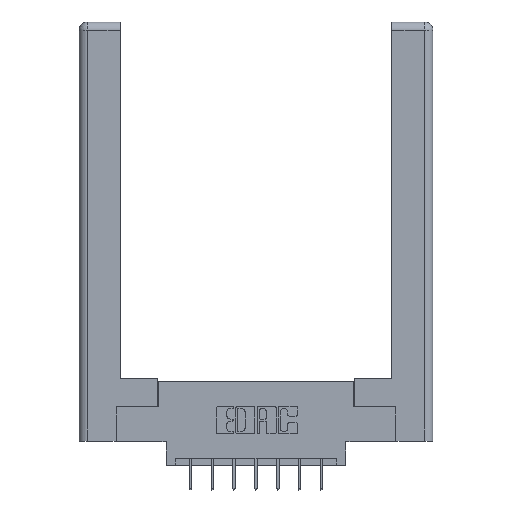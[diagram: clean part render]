
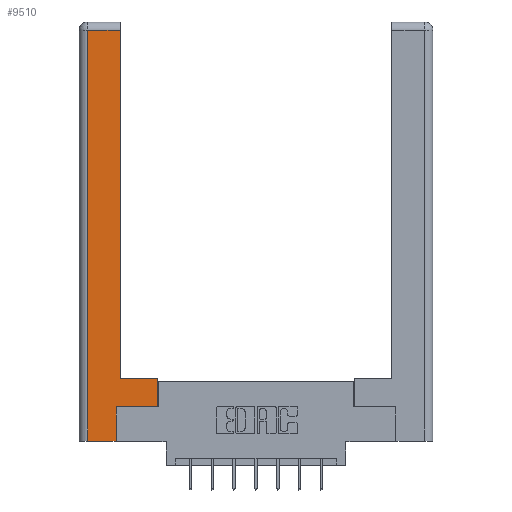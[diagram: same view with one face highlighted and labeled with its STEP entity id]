
A CAD part, top view. The second image highlights one B-rep face of the part: STEP entity #9510.
In plain terms, the highlighted planar face has unit normal (0, 0, 1).
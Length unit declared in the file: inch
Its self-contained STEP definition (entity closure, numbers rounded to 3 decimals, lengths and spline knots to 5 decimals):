
#22 = VECTOR ( 'NONE', #7003, 39.37008 ) ;
#182 = EDGE_CURVE ( 'NONE', #4637, #9045, #12069, .T. ) ;
#260 = EDGE_CURVE ( 'NONE', #9697, #6665, #2271, .T. ) ;
#274 = DIRECTION ( 'NONE',  ( 1., 0., 0. ) ) ;
#299 = DIRECTION ( 'NONE',  ( -1., 0., 0. ) ) ;
#448 = CARTESIAN_POINT ( 'NONE',  ( 0.265, 0., 0. ) ) ;
#798 = LINE ( 'NONE', #4582, #10724 ) ;
#1360 = EDGE_CURVE ( 'NONE', #6665, #6210, #3975, .T. ) ;
#1703 = CARTESIAN_POINT ( 'NONE',  ( 0.565, 0.245, 0. ) ) ;
#2098 = CARTESIAN_POINT ( 'NONE',  ( 0., 0., 0. ) ) ;
#2271 = LINE ( 'NONE', #12100, #2762 ) ;
#2762 = VECTOR ( 'NONE', #274, 39.37008 ) ;
#2773 = DIRECTION ( 'NONE',  ( 0., 1., 0. ) ) ;
#2779 = ORIENTED_EDGE ( 'NONE', *, *, #182, .T. ) ;
#3122 = PLANE ( 'NONE',  #3259 ) ;
#3156 = ORIENTED_EDGE ( 'NONE', *, *, #4292, .T. ) ;
#3259 = AXIS2_PLACEMENT_3D ( 'NONE', #2098, #9182, #299 ) ;
#3463 = VERTEX_POINT ( 'NONE', #12084 ) ;
#3745 = FACE_OUTER_BOUND ( 'NONE', #10373, .T. ) ;
#3843 = EDGE_CURVE ( 'NONE', #6210, #11809, #7038, .T. ) ;
#3860 = CARTESIAN_POINT ( 'NONE',  ( 0.565, 0.45, 0. ) ) ;
#3975 = LINE ( 'NONE', #12767, #9234 ) ;
#4292 = EDGE_CURVE ( 'NONE', #3463, #9697, #7168, .T. ) ;
#4330 = EDGE_CURVE ( 'NONE', #9292, #3463, #798, .T. ) ;
#4582 = CARTESIAN_POINT ( 'NONE',  ( 0.0615, 2.94, 0. ) ) ;
#4637 = VERTEX_POINT ( 'NONE', #3860 ) ;
#4691 = EDGE_CURVE ( 'NONE', #11809, #4637, #11178, .T. ) ;
#5082 = EDGE_CURVE ( 'NONE', #9045, #9292, #5582, .T. ) ;
#5582 = LINE ( 'NONE', #11931, #22 ) ;
#5899 = CARTESIAN_POINT ( 'NONE',  ( 0.565, 0.45, 0. ) ) ;
#6210 = VERTEX_POINT ( 'NONE', #10511 ) ;
#6430 = CARTESIAN_POINT ( 'NONE',  ( 0.0615, 0., 0. ) ) ;
#6665 = VERTEX_POINT ( 'NONE', #448 ) ;
#6757 = ORIENTED_EDGE ( 'NONE', *, *, #4691, .T. ) ;
#7003 = DIRECTION ( 'NONE',  ( 0., 1., 0. ) ) ;
#7019 = CARTESIAN_POINT ( 'NONE',  ( 0.565, 0.245, 0. ) ) ;
#7038 = LINE ( 'NONE', #1703, #11990 ) ;
#7168 = LINE ( 'NONE', #6430, #12421 ) ;
#7265 = ORIENTED_EDGE ( 'NONE', *, *, #4330, .T. ) ;
#7311 = VECTOR ( 'NONE', #11728, 39.37008 ) ;
#7432 = DIRECTION ( 'NONE',  ( -1., 0., 0. ) ) ;
#8430 = DIRECTION ( 'NONE',  ( 0., -1., 0. ) ) ;
#9045 = VERTEX_POINT ( 'NONE', #10155 ) ;
#9113 = DIRECTION ( 'NONE',  ( -1., 0., 0. ) ) ;
#9161 = ORIENTED_EDGE ( 'NONE', *, *, #260, .T. ) ;
#9182 = DIRECTION ( 'NONE',  ( 0., 0., -1. ) ) ;
#9234 = VECTOR ( 'NONE', #2773, 39.37008 ) ;
#9292 = VERTEX_POINT ( 'NONE', #9799 ) ;
#9510 = ADVANCED_FACE ( 'NONE', ( #3745 ), #3122, .F. ) ;
#9531 = ORIENTED_EDGE ( 'NONE', *, *, #5082, .T. ) ;
#9697 = VERTEX_POINT ( 'NONE', #10393 ) ;
#9799 = CARTESIAN_POINT ( 'NONE',  ( 0.295, 2.94, 0. ) ) ;
#10155 = CARTESIAN_POINT ( 'NONE',  ( 0.295, 0.45, 0. ) ) ;
#10373 = EDGE_LOOP ( 'NONE', ( #9531, #7265, #3156, #9161, #11721, #11979, #6757, #2779 ) ) ;
#10393 = CARTESIAN_POINT ( 'NONE',  ( 0.0615, 0., 0. ) ) ;
#10511 = CARTESIAN_POINT ( 'NONE',  ( 0.265, 0.245, 0. ) ) ;
#10724 = VECTOR ( 'NONE', #7432, 39.37008 ) ;
#11178 = LINE ( 'NONE', #5899, #7311 ) ;
#11223 = CARTESIAN_POINT ( 'NONE',  ( 0.295, 0.45, 0. ) ) ;
#11436 = VECTOR ( 'NONE', #9113, 39.37008 ) ;
#11590 = DIRECTION ( 'NONE',  ( 1., 0., 0. ) ) ;
#11721 = ORIENTED_EDGE ( 'NONE', *, *, #1360, .T. ) ;
#11728 = DIRECTION ( 'NONE',  ( 0., 1., 0. ) ) ;
#11809 = VERTEX_POINT ( 'NONE', #7019 ) ;
#11931 = CARTESIAN_POINT ( 'NONE',  ( 0.295, 3., 0. ) ) ;
#11979 = ORIENTED_EDGE ( 'NONE', *, *, #3843, .T. ) ;
#11990 = VECTOR ( 'NONE', #11590, 39.37008 ) ;
#12069 = LINE ( 'NONE', #11223, #11436 ) ;
#12084 = CARTESIAN_POINT ( 'NONE',  ( 0.0615, 2.94, 0. ) ) ;
#12100 = CARTESIAN_POINT ( 'NONE',  ( 0.265, 0., 0. ) ) ;
#12421 = VECTOR ( 'NONE', #8430, 39.37008 ) ;
#12767 = CARTESIAN_POINT ( 'NONE',  ( 0.265, 0.245, 0. ) ) ;
